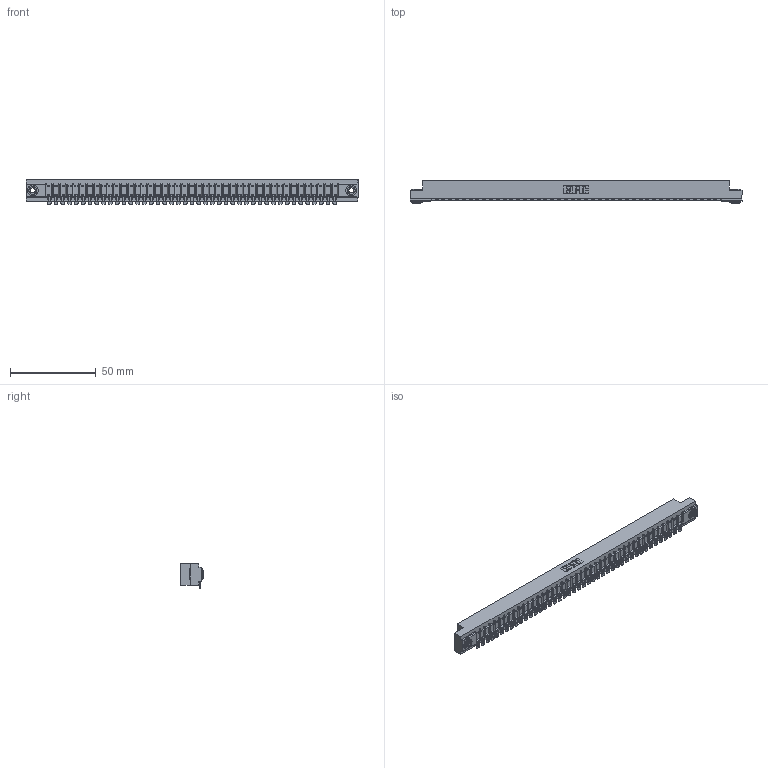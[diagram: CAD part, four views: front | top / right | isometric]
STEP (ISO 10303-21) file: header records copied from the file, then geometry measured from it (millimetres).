
FILE_DESCRIPTION (( 'STEP AP203' ), '1' );
FILE_NAME ('307-043-554-103.STEP', '2018-08-06T00:58:38', ( '' ), ( '' ), 'SwSTEP 2.0', 'SolidWorks 2016', '' );
FILE_SCHEMA (( 'CONFIG_CONTROL_DESIGN' ));
Length unit declared in the file: inch
Products named in the file (4): 307 Part_.156 Dia Mounting Holes; 307-290-002_554; 345-250-002_345-250-002-102; 307-043-554-103
Assembly tree (46 placements, depth 2):
  307-043-554-103
    307 Part_.156 Dia Mounting Holes
    307-290-002_554  x43
    345-250-002_345-250-002-102  x2
Bounding box: 193.4 x 13.36 x 14.52 mm (x, y, z)
Volume: 20720 mm3; surface area: 26489.1 mm2
Topology: 46 solids, 46 shells, 3697 faces, 11314 edges, 7420 vertices
Faces by surface type: plane 2072, cylinder 1529, sphere 88, cone 8
Entity records: 38770 total; most frequent: CARTESIAN_POINT 6519, ORIENTED_EDGE 6500, DIRECTION 6354, EDGE_CURVE 3250, LINE 2476, VECTOR 2476, VERTEX_POINT 2104, AXIS2_PLACEMENT_3D 1939
